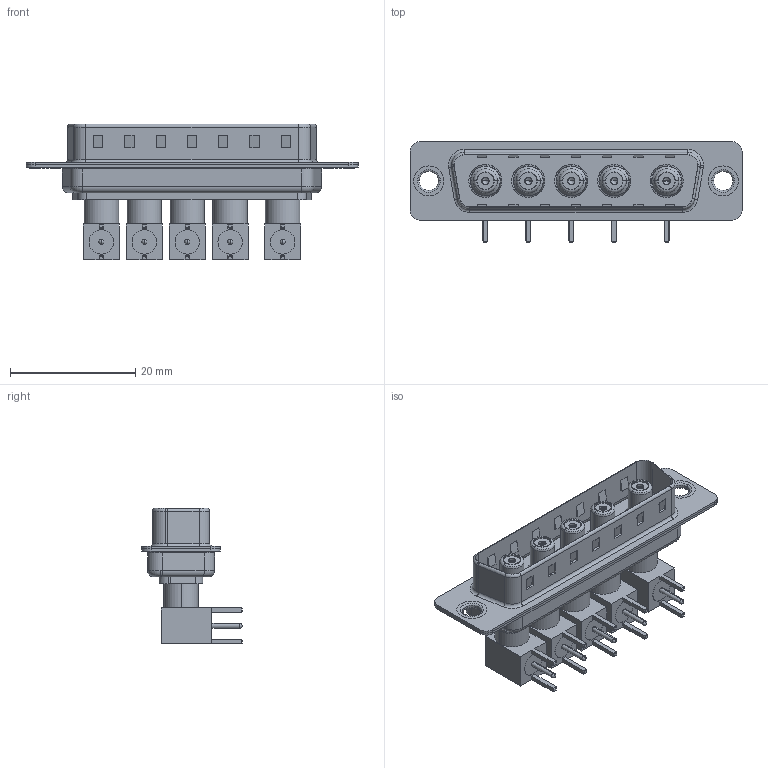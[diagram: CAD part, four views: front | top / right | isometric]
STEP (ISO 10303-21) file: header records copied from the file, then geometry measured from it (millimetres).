
FILE_DESCRIPTION (( 'STEP AP203' ), '1' );
FILE_NAME ('629-5W5-240-5N1.STEP', '2022-05-07T05:36:18', ( '' ), ( '' ), 'SwSTEP 2.0', 'SolidWorks 2020', '' );
FILE_SCHEMA (( 'CONFIG_CONTROL_DESIGN' ));
Length unit declared in the file: millimetre
Products named in the file (17): RA Back Shell; 629Combo Thru Hole Rivet; Locking Collar; Insulator Socket 2; Co-Ax Jack Assy_RA; Insulator Socket; 629Combo Shell Rear_25 Contacts; 629Combo Shell Front_25 Contacts; Socket_RA; 629Combo Housing_5W5; Co-Ax Jack_RA PC Tail; Insulator RA Pin; 629-5W5-240-5N1
Assembly tree (45 placements, depth 3):
  629-5W5-240-5N1
    629Combo Housing_5W5
    629Combo Shell Rear_25 Contacts
    629Combo Shell Front_25 Contacts
    629Combo Thru Hole Rivet  x2
    Co-Ax Jack Assy_RA
      Co-Ax Jack_RA PC Tail
      Insulator Socket
      Insulator Socket 2
      Locking Collar
      Socket_RA
      RA Back Shell
      Insulator RA Pin
    Co-Ax Jack Assy_RA
      Co-Ax Jack_RA PC Tail
      Insulator Socket
      Insulator Socket 2
      Locking Collar
      Socket_RA
      RA Back Shell
      Insulator RA Pin
    Co-Ax Jack Assy_RA
      Co-Ax Jack_RA PC Tail
      Insulator Socket
      Insulator Socket 2
      Locking Collar
      Socket_RA
      RA Back Shell
      Insulator RA Pin
    Co-Ax Jack Assy_RA
      Co-Ax Jack_RA PC Tail
      Insulator Socket
      Insulator Socket 2
      Locking Collar
      Socket_RA
      RA Back Shell
      Insulator RA Pin
    Co-Ax Jack Assy_RA
      Co-Ax Jack_RA PC Tail
      Insulator Socket
      Insulator Socket 2
      Locking Collar
      Socket_RA
      RA Back Shell
      Insulator RA Pin
Bounding box: 53.05 x 16 x 21.71 mm (x, y, z)
Volume: 4066.4 mm3; surface area: 11223.6 mm2
Topology: 40 solids, 40 shells, 1110 faces, 2600 edges, 1611 vertices
Faces by surface type: cylinder 456, plane 456, cone 95, torus 88, sphere 10, bspline 5
Entity records: 17744 total; most frequent: CARTESIAN_POINT 2797, DIRECTION 2777, ORIENTED_EDGE 2432, EDGE_CURVE 1216, AXIS2_PLACEMENT_3D 1040, VERTEX_POINT 765, VECTOR 697, LINE 697
